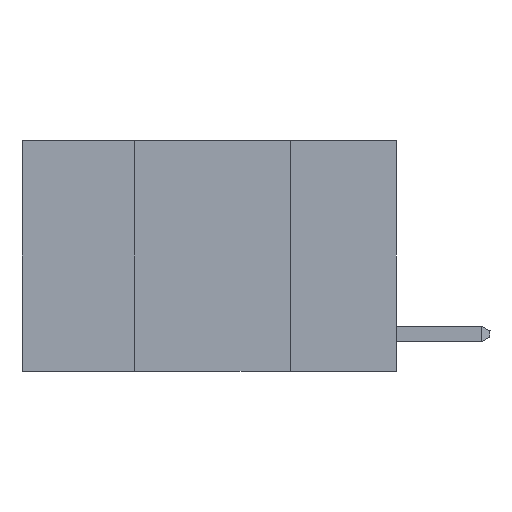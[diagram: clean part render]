
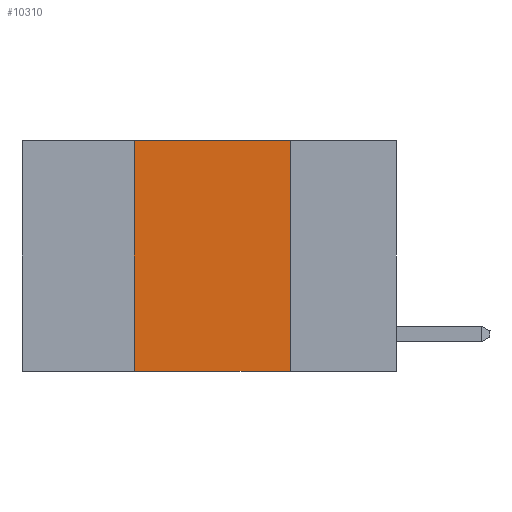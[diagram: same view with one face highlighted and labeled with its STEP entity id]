
A CAD part, left-side view. The second image highlights one B-rep face of the part: STEP entity #10310.
In plain terms, the highlighted planar face has unit normal (-1, 0, 0).
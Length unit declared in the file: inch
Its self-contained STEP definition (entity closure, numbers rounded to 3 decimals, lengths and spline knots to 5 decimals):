
#141 = VERTEX_POINT ( 'NONE', #2487 ) ;
#760 = DIRECTION ( 'NONE',  ( 0., -1., 0. ) ) ;
#970 = LINE ( 'NONE', #10084, #3216 ) ;
#1408 = EDGE_LOOP ( 'NONE', ( #5438, #9500, #12096, #4438 ) ) ;
#2124 = EDGE_CURVE ( 'NONE', #5811, #141, #3943, .T. ) ;
#2163 = AXIS2_PLACEMENT_3D ( 'NONE', #11901, #9960, #11856 ) ;
#2487 = CARTESIAN_POINT ( 'NONE',  ( 0., 0.42, 0. ) ) ;
#2660 = CARTESIAN_POINT ( 'NONE',  ( 0., 0.6, 0. ) ) ;
#3216 = VECTOR ( 'NONE', #10897, 39.37008 ) ;
#3314 = CARTESIAN_POINT ( 'NONE',  ( 0., 0.42, 0. ) ) ;
#3361 = VECTOR ( 'NONE', #7932, 39.37008 ) ;
#3943 = LINE ( 'NONE', #3314, #3361 ) ;
#4182 = VERTEX_POINT ( 'NONE', #5237 ) ;
#4256 = VECTOR ( 'NONE', #5362, 39.37008 ) ;
#4438 = ORIENTED_EDGE ( 'NONE', *, *, #7391, .T. ) ;
#5237 = CARTESIAN_POINT ( 'NONE',  ( 0., 0.17, 0. ) ) ;
#5362 = DIRECTION ( 'NONE',  ( 0., -1., 0. ) ) ;
#5421 = LINE ( 'NONE', #7182, #4256 ) ;
#5438 = ORIENTED_EDGE ( 'NONE', *, *, #8621, .F. ) ;
#5811 = VERTEX_POINT ( 'NONE', #6040 ) ;
#6040 = CARTESIAN_POINT ( 'NONE',  ( 0., 0.42, -0.37 ) ) ;
#6425 = LINE ( 'NONE', #2660, #11677 ) ;
#6895 = CARTESIAN_POINT ( 'NONE',  ( 0., 0.17, -0.37 ) ) ;
#7182 = CARTESIAN_POINT ( 'NONE',  ( 0., 0.6, -0.37 ) ) ;
#7391 = EDGE_CURVE ( 'NONE', #5811, #10617, #5421, .T. ) ;
#7932 = DIRECTION ( 'NONE',  ( 0., 0., 1. ) ) ;
#8131 = PLANE ( 'NONE',  #2163 ) ;
#8621 = EDGE_CURVE ( 'NONE', #4182, #10617, #970, .T. ) ;
#9500 = ORIENTED_EDGE ( 'NONE', *, *, #11936, .F. ) ;
#9960 = DIRECTION ( 'NONE',  ( 1., 0., 0. ) ) ;
#10084 = CARTESIAN_POINT ( 'NONE',  ( 0., 0.17, 0. ) ) ;
#10310 = ADVANCED_FACE ( 'NONE', ( #11904 ), #8131, .F. ) ;
#10617 = VERTEX_POINT ( 'NONE', #6895 ) ;
#10897 = DIRECTION ( 'NONE',  ( 0., 0., -1. ) ) ;
#11677 = VECTOR ( 'NONE', #760, 39.37008 ) ;
#11856 = DIRECTION ( 'NONE',  ( 0., 0., -1. ) ) ;
#11901 = CARTESIAN_POINT ( 'NONE',  ( 0., 0.6, 0. ) ) ;
#11904 = FACE_OUTER_BOUND ( 'NONE', #1408, .T. ) ;
#11936 = EDGE_CURVE ( 'NONE', #141, #4182, #6425, .T. ) ;
#12096 = ORIENTED_EDGE ( 'NONE', *, *, #2124, .F. ) ;
